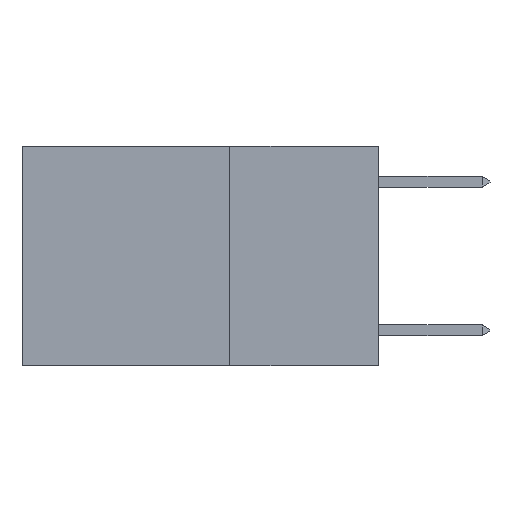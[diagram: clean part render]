
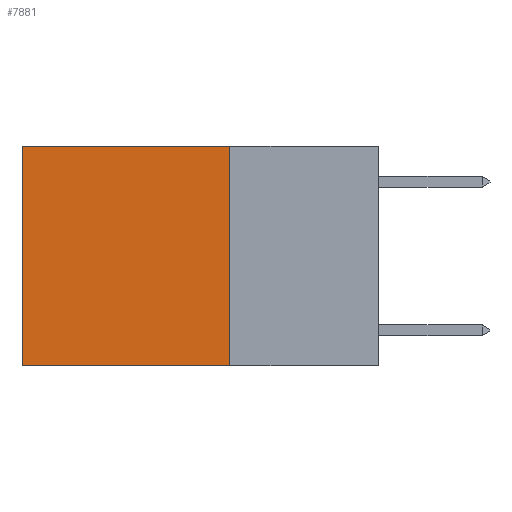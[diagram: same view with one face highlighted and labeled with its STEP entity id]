
A CAD part, left-side view. The second image highlights one B-rep face of the part: STEP entity #7881.
In plain terms, the highlighted planar face has unit normal (-1, 0, 0).
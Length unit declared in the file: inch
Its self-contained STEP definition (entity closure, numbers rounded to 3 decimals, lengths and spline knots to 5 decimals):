
#223 = CARTESIAN_POINT ( 'NONE',  ( 0.2625, 0.6, 0. ) ) ;
#335 = CARTESIAN_POINT ( 'NONE',  ( 0.2625, 0.25, -0.37 ) ) ;
#733 = VERTEX_POINT ( 'NONE', #2637 ) ;
#787 = CARTESIAN_POINT ( 'NONE',  ( 0.2625, 0.25, 0. ) ) ;
#976 = FACE_OUTER_BOUND ( 'NONE', #7581, .T. ) ;
#1409 = ORIENTED_EDGE ( 'NONE', *, *, #8023, .T. ) ;
#1744 = DIRECTION ( 'NONE',  ( 1., 0., 0. ) ) ;
#1787 = PLANE ( 'NONE',  #6543 ) ;
#1930 = VERTEX_POINT ( 'NONE', #7062 ) ;
#2362 = EDGE_CURVE ( 'NONE', #1930, #5929, #3694, .T. ) ;
#2588 = CARTESIAN_POINT ( 'NONE',  ( 0.2625, 0.25, 0. ) ) ;
#2609 = CARTESIAN_POINT ( 'NONE',  ( 0.2625, 0.6, -0.37 ) ) ;
#2637 = CARTESIAN_POINT ( 'NONE',  ( 0.2625, 0.25, -0.37 ) ) ;
#2931 = ORIENTED_EDGE ( 'NONE', *, *, #7111, .F. ) ;
#2987 = LINE ( 'NONE', #335, #4017 ) ;
#3694 = LINE ( 'NONE', #223, #7448 ) ;
#4017 = VECTOR ( 'NONE', #7746, 39.37008 ) ;
#4297 = LINE ( 'NONE', #787, #5641 ) ;
#4491 = DIRECTION ( 'NONE',  ( 0., 0., -1. ) ) ;
#4662 = LINE ( 'NONE', #7306, #8275 ) ;
#5294 = ORIENTED_EDGE ( 'NONE', *, *, #8665, .F. ) ;
#5641 = VECTOR ( 'NONE', #7690, 39.37008 ) ;
#5929 = VERTEX_POINT ( 'NONE', #2609 ) ;
#6543 = AXIS2_PLACEMENT_3D ( 'NONE', #7212, #1744, #4491 ) ;
#6634 = DIRECTION ( 'NONE',  ( 0., 1., 0. ) ) ;
#6787 = VERTEX_POINT ( 'NONE', #2588 ) ;
#7054 = DIRECTION ( 'NONE',  ( 0., 0., -1. ) ) ;
#7062 = CARTESIAN_POINT ( 'NONE',  ( 0.2625, 0.6, 0. ) ) ;
#7111 = EDGE_CURVE ( 'NONE', #733, #5929, #2987, .T. ) ;
#7212 = CARTESIAN_POINT ( 'NONE',  ( 0.2625, 0.25, 0. ) ) ;
#7306 = CARTESIAN_POINT ( 'NONE',  ( 0.2625, 0.25, 0. ) ) ;
#7448 = VECTOR ( 'NONE', #7054, 39.37008 ) ;
#7581 = EDGE_LOOP ( 'NONE', ( #8759, #2931, #5294, #1409 ) ) ;
#7690 = DIRECTION ( 'NONE',  ( 0., 0., -1. ) ) ;
#7746 = DIRECTION ( 'NONE',  ( 0., 1., 0. ) ) ;
#7881 = ADVANCED_FACE ( 'NONE', ( #976 ), #1787, .F. ) ;
#8023 = EDGE_CURVE ( 'NONE', #6787, #1930, #4662, .T. ) ;
#8275 = VECTOR ( 'NONE', #6634, 39.37008 ) ;
#8665 = EDGE_CURVE ( 'NONE', #6787, #733, #4297, .T. ) ;
#8759 = ORIENTED_EDGE ( 'NONE', *, *, #2362, .T. ) ;
